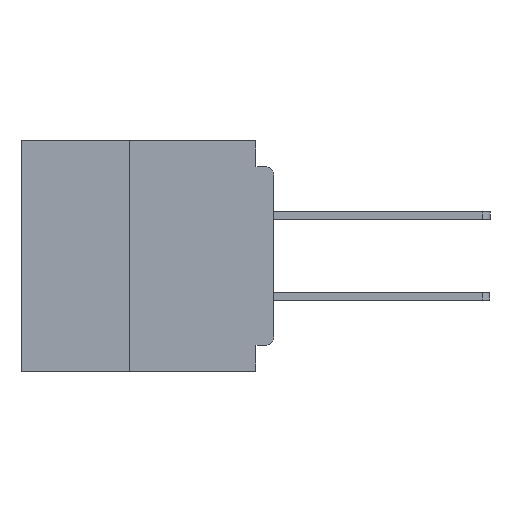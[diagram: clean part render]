
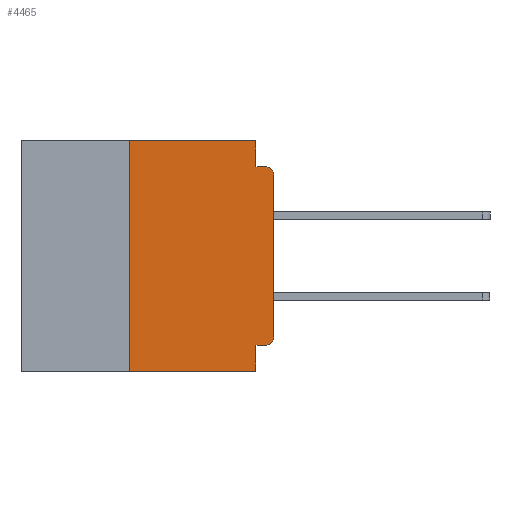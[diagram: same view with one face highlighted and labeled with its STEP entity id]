
A CAD part, left-side view. The second image highlights one B-rep face of the part: STEP entity #4465.
In plain terms, the highlighted planar face has unit normal (-1, 0, 0).
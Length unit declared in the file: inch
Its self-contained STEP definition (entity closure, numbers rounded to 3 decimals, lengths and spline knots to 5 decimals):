
#366 = ORIENTED_EDGE ( 'NONE', *, *, #34774, .T. ) ;
#592 = LINE ( 'NONE', #12301, #18340 ) ;
#1224 = VERTEX_POINT ( 'NONE', #30227 ) ;
#2118 = DIRECTION ( 'NONE',  ( 0., -1., 0. ) ) ;
#2181 = VERTEX_POINT ( 'NONE', #13773 ) ;
#4003 = ORIENTED_EDGE ( 'NONE', *, *, #17388, .F. ) ;
#4464 = ORIENTED_EDGE ( 'NONE', *, *, #11114, .T. ) ;
#4465 = ADVANCED_FACE ( 'NONE', ( #38545 ), #5591, .F. ) ;
#4506 = ORIENTED_EDGE ( 'NONE', *, *, #21343, .F. ) ;
#5194 = EDGE_LOOP ( 'NONE', ( #4464, #24759, #39659, #40838, #12902, #33109, #366, #4506, #4003, #31933 ) ) ;
#5331 = CARTESIAN_POINT ( 'NONE',  ( 0., 0., -0.06 ) ) ;
#5591 = PLANE ( 'NONE',  #18818 ) ;
#5826 = CARTESIAN_POINT ( 'NONE',  ( 0., 0.437, 0. ) ) ;
#6047 = LINE ( 'NONE', #33791, #32094 ) ;
#6392 = CARTESIAN_POINT ( 'NONE',  ( 0., 0.031, 0. ) ) ;
#6840 = VERTEX_POINT ( 'NONE', #39138 ) ;
#7619 = CARTESIAN_POINT ( 'NONE',  ( 0., 0.25, 0. ) ) ;
#9181 = VECTOR ( 'NONE', #16017, 39.37008 ) ;
#9188 = DIRECTION ( 'NONE',  ( 1., 0., 0. ) ) ;
#9281 = EDGE_CURVE ( 'NONE', #24237, #6840, #13226, .T. ) ;
#11114 = EDGE_CURVE ( 'NONE', #15374, #24237, #25133, .T. ) ;
#12188 = DIRECTION ( 'NONE',  ( -1., 0., 0. ) ) ;
#12301 = CARTESIAN_POINT ( 'NONE',  ( 0., 0., -0.045 ) ) ;
#12590 = EDGE_CURVE ( 'NONE', #1224, #6840, #592, .T. ) ;
#12727 = VECTOR ( 'NONE', #28249, 39.37008 ) ;
#12902 = ORIENTED_EDGE ( 'NONE', *, *, #29763, .F. ) ;
#13226 = CIRCLE ( 'NONE', #20763, 0.015 ) ;
#13548 = DIRECTION ( 'NONE',  ( 0., 0., -1. ) ) ;
#13595 = EDGE_CURVE ( 'NONE', #17587, #21092, #31534, .T. ) ;
#13773 = CARTESIAN_POINT ( 'NONE',  ( 0., 0.031, -0.4 ) ) ;
#14287 = CARTESIAN_POINT ( 'NONE',  ( 0., 0.25, -0.4 ) ) ;
#15337 = EDGE_CURVE ( 'NONE', #31511, #1224, #24783, .T. ) ;
#15374 = VERTEX_POINT ( 'NONE', #24214 ) ;
#15418 = VECTOR ( 'NONE', #13548, 39.37008 ) ;
#15879 = CARTESIAN_POINT ( 'NONE',  ( 0., 0., -0.355 ) ) ;
#16017 = DIRECTION ( 'NONE',  ( 0., 1., 0. ) ) ;
#16145 = DIRECTION ( 'NONE',  ( 0., 0., -1. ) ) ;
#16733 = VECTOR ( 'NONE', #2118, 39.37008 ) ;
#17388 = EDGE_CURVE ( 'NONE', #18982, #36028, #29132, .T. ) ;
#17587 = VERTEX_POINT ( 'NONE', #14287 ) ;
#17746 = DIRECTION ( 'NONE',  ( -1., 0., 0. ) ) ;
#18340 = VECTOR ( 'NONE', #44124, 39.37008 ) ;
#18818 = AXIS2_PLACEMENT_3D ( 'NONE', #23258, #9188, #33947 ) ;
#18982 = VERTEX_POINT ( 'NONE', #27457 ) ;
#20763 = AXIS2_PLACEMENT_3D ( 'NONE', #38942, #17746, #42445 ) ;
#21092 = VERTEX_POINT ( 'NONE', #7619 ) ;
#21343 = EDGE_CURVE ( 'NONE', #36028, #2181, #6047, .T. ) ;
#22748 = VECTOR ( 'NONE', #34333, 39.37008 ) ;
#23258 = CARTESIAN_POINT ( 'NONE',  ( 0., 0.437, 0. ) ) ;
#23389 = CARTESIAN_POINT ( 'NONE',  ( 0., 0.437, -0.4 ) ) ;
#24214 = CARTESIAN_POINT ( 'NONE',  ( 0., 0., -0.34 ) ) ;
#24237 = VERTEX_POINT ( 'NONE', #5331 ) ;
#24641 = CIRCLE ( 'NONE', #24646, 0.015 ) ;
#24646 = AXIS2_PLACEMENT_3D ( 'NONE', #33411, #12188, #36963 ) ;
#24759 = ORIENTED_EDGE ( 'NONE', *, *, #9281, .T. ) ;
#24783 = LINE ( 'NONE', #6392, #15418 ) ;
#25133 = LINE ( 'NONE', #39490, #33469 ) ;
#27457 = CARTESIAN_POINT ( 'NONE',  ( 0., 0.015, -0.355 ) ) ;
#28249 = DIRECTION ( 'NONE',  ( 0., 0., 1. ) ) ;
#29132 = LINE ( 'NONE', #15879, #9181 ) ;
#29763 = EDGE_CURVE ( 'NONE', #21092, #31511, #32149, .T. ) ;
#30227 = CARTESIAN_POINT ( 'NONE',  ( 0., 0.031, -0.045 ) ) ;
#31511 = VERTEX_POINT ( 'NONE', #36464 ) ;
#31534 = LINE ( 'NONE', #45827, #12727 ) ;
#31933 = ORIENTED_EDGE ( 'NONE', *, *, #32879, .T. ) ;
#32094 = VECTOR ( 'NONE', #16145, 39.37008 ) ;
#32149 = LINE ( 'NONE', #5826, #22748 ) ;
#32879 = EDGE_CURVE ( 'NONE', #18982, #15374, #24641, .T. ) ;
#33109 = ORIENTED_EDGE ( 'NONE', *, *, #13595, .F. ) ;
#33411 = CARTESIAN_POINT ( 'NONE',  ( 0., 0.015, -0.34 ) ) ;
#33469 = VECTOR ( 'NONE', #43015, 39.37008 ) ;
#33791 = CARTESIAN_POINT ( 'NONE',  ( 0., 0.031, -0.4 ) ) ;
#33947 = DIRECTION ( 'NONE',  ( 0., 0., -1. ) ) ;
#34333 = DIRECTION ( 'NONE',  ( 0., -1., 0. ) ) ;
#34774 = EDGE_CURVE ( 'NONE', #17587, #2181, #35555, .T. ) ;
#35555 = LINE ( 'NONE', #23389, #16733 ) ;
#36028 = VERTEX_POINT ( 'NONE', #37232 ) ;
#36464 = CARTESIAN_POINT ( 'NONE',  ( 0., 0.031, 0. ) ) ;
#36963 = DIRECTION ( 'NONE',  ( 0., 0., -1. ) ) ;
#37232 = CARTESIAN_POINT ( 'NONE',  ( 0., 0.031, -0.355 ) ) ;
#38545 = FACE_OUTER_BOUND ( 'NONE', #5194, .T. ) ;
#38942 = CARTESIAN_POINT ( 'NONE',  ( 0., 0.015, -0.06 ) ) ;
#39138 = CARTESIAN_POINT ( 'NONE',  ( 0., 0.015, -0.045 ) ) ;
#39490 = CARTESIAN_POINT ( 'NONE',  ( 0., 0., 0. ) ) ;
#39659 = ORIENTED_EDGE ( 'NONE', *, *, #12590, .F. ) ;
#40838 = ORIENTED_EDGE ( 'NONE', *, *, #15337, .F. ) ;
#42445 = DIRECTION ( 'NONE',  ( 0., 0., -1. ) ) ;
#43015 = DIRECTION ( 'NONE',  ( 0., 0., 1. ) ) ;
#44124 = DIRECTION ( 'NONE',  ( 0., -1., 0. ) ) ;
#45827 = CARTESIAN_POINT ( 'NONE',  ( 0., 0.25, -0.4 ) ) ;
